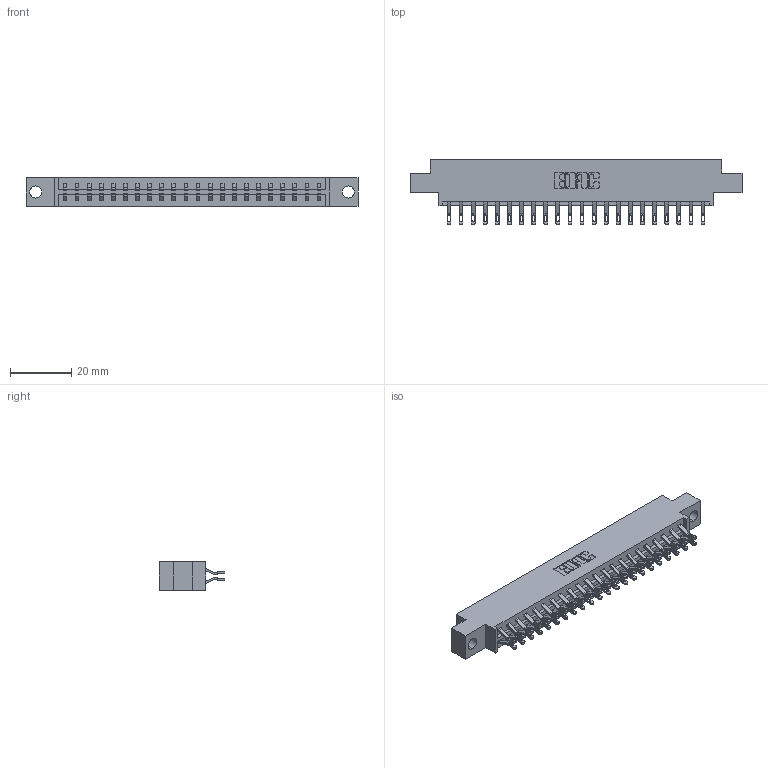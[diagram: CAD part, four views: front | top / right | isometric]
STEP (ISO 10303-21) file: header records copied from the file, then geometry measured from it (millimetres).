
FILE_DESCRIPTION (( 'STEP AP203' ), '1' );
FILE_NAME ('833-044-555-804.STEP', '2020-06-04T01:48:02', ( '' ), ( '' ), 'SwSTEP 2.0', 'SolidWorks 2020', '' );
FILE_SCHEMA (( 'CONFIG_CONTROL_DESIGN' ));
Length unit declared in the file: inch
Products named in the file (3): 833-044-555-804; 345-292-001_555 Tail; 833 Part_Offset - .156 Dia - TH
Assembly tree (45 placements, depth 2):
  833-044-555-804
    833 Part_Offset - .156 Dia - TH
    345-292-001_555 Tail  x44
Bounding box: 108.71 x 21.47 x 9.4 mm (x, y, z)
Volume: 10723.8 mm3; surface area: 12960.9 mm2
Topology: 45 solids, 45 shells, 2670 faces, 8375 edges, 5582 vertices
Faces by surface type: plane 1570, cylinder 1100
Entity records: 17201 total; most frequent: CARTESIAN_POINT 2912, ORIENTED_EDGE 2818, DIRECTION 2493, EDGE_CURVE 1409, LINE 1261, VECTOR 1261, VERTEX_POINT 938, AXIS2_PLACEMENT_3D 616
